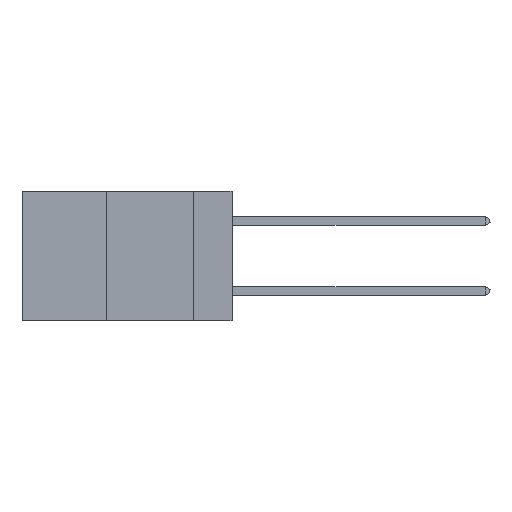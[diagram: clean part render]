
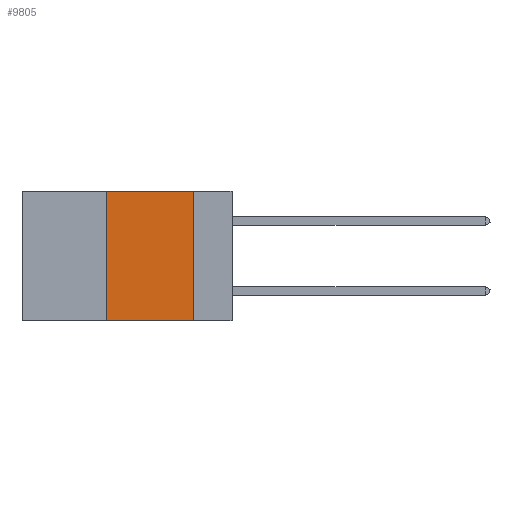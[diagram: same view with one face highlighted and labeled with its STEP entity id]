
A CAD part, left-side view. The second image highlights one B-rep face of the part: STEP entity #9805.
In plain terms, the highlighted planar face has unit normal (-1, 0, 0).
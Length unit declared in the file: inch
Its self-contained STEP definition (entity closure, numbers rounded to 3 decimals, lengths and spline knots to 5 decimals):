
#1178 = VERTEX_POINT ( 'NONE', #9226 ) ;
#1424 = LINE ( 'NONE', #16713, #21498 ) ;
#1585 = DIRECTION ( 'NONE',  ( 1., 0., 0. ) ) ;
#3202 = DIRECTION ( 'NONE',  ( 0., 0., -1. ) ) ;
#3221 = CARTESIAN_POINT ( 'NONE',  ( 0., 0.6, 0. ) ) ;
#3286 = EDGE_CURVE ( 'NONE', #6309, #3328, #8203, .T. ) ;
#3328 = VERTEX_POINT ( 'NONE', #26347 ) ;
#3560 = VERTEX_POINT ( 'NONE', #8803 ) ;
#6309 = VERTEX_POINT ( 'NONE', #10190 ) ;
#6399 = EDGE_LOOP ( 'NONE', ( #9848, #18101, #26198, #33058 ) ) ;
#8203 = LINE ( 'NONE', #15866, #34354 ) ;
#8376 = EDGE_CURVE ( 'NONE', #1178, #6309, #33218, .T. ) ;
#8581 = DIRECTION ( 'NONE',  ( 0., -1., 0. ) ) ;
#8803 = CARTESIAN_POINT ( 'NONE',  ( 0., 0.11, -0.37 ) ) ;
#9226 = CARTESIAN_POINT ( 'NONE',  ( 0., 0.36, -0.37 ) ) ;
#9554 = DIRECTION ( 'NONE',  ( 0., 0., 1. ) ) ;
#9805 = ADVANCED_FACE ( 'NONE', ( #16308 ), #22454, .F. ) ;
#9848 = ORIENTED_EDGE ( 'NONE', *, *, #33368, .F. ) ;
#10190 = CARTESIAN_POINT ( 'NONE',  ( 0., 0.36, 0. ) ) ;
#11701 = VECTOR ( 'NONE', #9554, 39.37008 ) ;
#14537 = EDGE_CURVE ( 'NONE', #1178, #3560, #1424, .T. ) ;
#15866 = CARTESIAN_POINT ( 'NONE',  ( 0., 0.6, 0. ) ) ;
#16308 = FACE_OUTER_BOUND ( 'NONE', #6399, .T. ) ;
#16713 = CARTESIAN_POINT ( 'NONE',  ( 0., 0.6, -0.37 ) ) ;
#17552 = AXIS2_PLACEMENT_3D ( 'NONE', #3221, #1585, #30997 ) ;
#18101 = ORIENTED_EDGE ( 'NONE', *, *, #3286, .F. ) ;
#18343 = DIRECTION ( 'NONE',  ( 0., -1., 0. ) ) ;
#21089 = LINE ( 'NONE', #24430, #25741 ) ;
#21498 = VECTOR ( 'NONE', #8581, 39.37008 ) ;
#22454 = PLANE ( 'NONE',  #17552 ) ;
#24430 = CARTESIAN_POINT ( 'NONE',  ( 0., 0.11, 0. ) ) ;
#25741 = VECTOR ( 'NONE', #3202, 39.37008 ) ;
#26198 = ORIENTED_EDGE ( 'NONE', *, *, #8376, .F. ) ;
#26347 = CARTESIAN_POINT ( 'NONE',  ( 0., 0.11, 0. ) ) ;
#30997 = DIRECTION ( 'NONE',  ( 0., 0., -1. ) ) ;
#33058 = ORIENTED_EDGE ( 'NONE', *, *, #14537, .T. ) ;
#33218 = LINE ( 'NONE', #34265, #11701 ) ;
#33368 = EDGE_CURVE ( 'NONE', #3328, #3560, #21089, .T. ) ;
#34265 = CARTESIAN_POINT ( 'NONE',  ( 0., 0.36, 0. ) ) ;
#34354 = VECTOR ( 'NONE', #18343, 39.37008 ) ;
